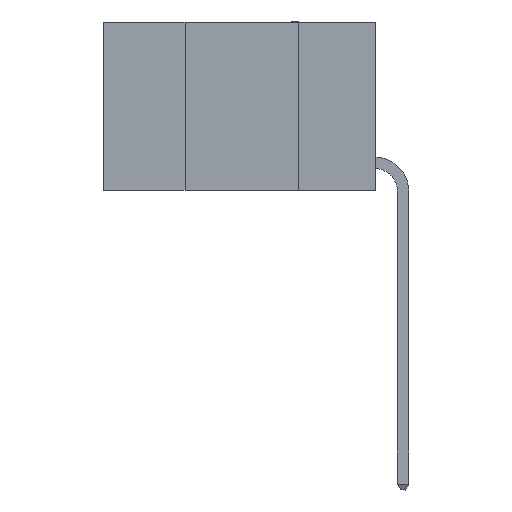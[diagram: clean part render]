
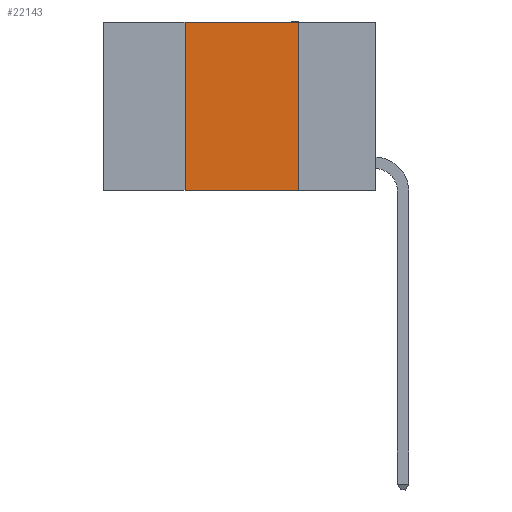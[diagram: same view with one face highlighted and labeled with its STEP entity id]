
A CAD part, left-side view. The second image highlights one B-rep face of the part: STEP entity #22143.
In plain terms, the highlighted planar face has unit normal (-1, 0, 0).
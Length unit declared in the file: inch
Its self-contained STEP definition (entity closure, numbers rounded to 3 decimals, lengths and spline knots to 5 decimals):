
#2203 = EDGE_CURVE ( 'NONE', #20575, #22809, #13826, .T. ) ;
#4812 = CARTESIAN_POINT ( 'NONE',  ( 0., 0.42, 0. ) ) ;
#4992 = AXIS2_PLACEMENT_3D ( 'NONE', #6134, #20291, #8188 ) ;
#5269 = EDGE_CURVE ( 'NONE', #9782, #22809, #9200, .T. ) ;
#5275 = DIRECTION ( 'NONE',  ( 0., -1., 0. ) ) ;
#5537 = EDGE_CURVE ( 'NONE', #21757, #20575, #17711, .T. ) ;
#5989 = CARTESIAN_POINT ( 'NONE',  ( 0., 0.6, 0. ) ) ;
#6134 = CARTESIAN_POINT ( 'NONE',  ( 0., 0.6, 0. ) ) ;
#6297 = VECTOR ( 'NONE', #10113, 39.37008 ) ;
#6633 = ORIENTED_EDGE ( 'NONE', *, *, #2203, .F. ) ;
#6638 = VECTOR ( 'NONE', #5275, 39.37008 ) ;
#7265 = ORIENTED_EDGE ( 'NONE', *, *, #5537, .F. ) ;
#8044 = CARTESIAN_POINT ( 'NONE',  ( 0., 0.42, 0. ) ) ;
#8188 = DIRECTION ( 'NONE',  ( 0., 0., -1. ) ) ;
#8435 = EDGE_LOOP ( 'NONE', ( #6633, #7265, #18038, #8546 ) ) ;
#8546 = ORIENTED_EDGE ( 'NONE', *, *, #5269, .T. ) ;
#9200 = LINE ( 'NONE', #15416, #6638 ) ;
#9782 = VERTEX_POINT ( 'NONE', #18108 ) ;
#10113 = DIRECTION ( 'NONE',  ( 0., -1., 0. ) ) ;
#12139 = DIRECTION ( 'NONE',  ( 0., 0., 1. ) ) ;
#12316 = FACE_OUTER_BOUND ( 'NONE', #8435, .T. ) ;
#12555 = LINE ( 'NONE', #8044, #22612 ) ;
#13199 = CARTESIAN_POINT ( 'NONE',  ( 0., 0.17, 0. ) ) ;
#13826 = LINE ( 'NONE', #24482, #23850 ) ;
#14228 = PLANE ( 'NONE',  #4992 ) ;
#15416 = CARTESIAN_POINT ( 'NONE',  ( 0., 0.6, -0.37 ) ) ;
#16476 = DIRECTION ( 'NONE',  ( 0., 0., -1. ) ) ;
#16860 = EDGE_CURVE ( 'NONE', #9782, #21757, #12555, .T. ) ;
#17711 = LINE ( 'NONE', #5989, #6297 ) ;
#18038 = ORIENTED_EDGE ( 'NONE', *, *, #16860, .F. ) ;
#18108 = CARTESIAN_POINT ( 'NONE',  ( 0., 0.42, -0.37 ) ) ;
#20291 = DIRECTION ( 'NONE',  ( 1., 0., 0. ) ) ;
#20575 = VERTEX_POINT ( 'NONE', #13199 ) ;
#21757 = VERTEX_POINT ( 'NONE', #4812 ) ;
#22143 = ADVANCED_FACE ( 'NONE', ( #12316 ), #14228, .F. ) ;
#22444 = CARTESIAN_POINT ( 'NONE',  ( 0., 0.17, -0.37 ) ) ;
#22612 = VECTOR ( 'NONE', #12139, 39.37008 ) ;
#22809 = VERTEX_POINT ( 'NONE', #22444 ) ;
#23850 = VECTOR ( 'NONE', #16476, 39.37008 ) ;
#24482 = CARTESIAN_POINT ( 'NONE',  ( 0., 0.17, 0. ) ) ;
